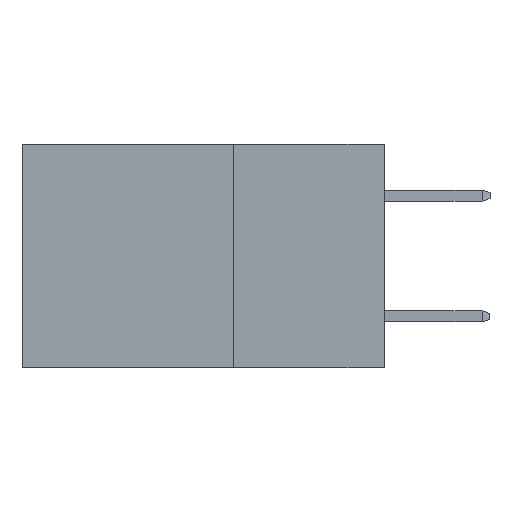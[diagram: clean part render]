
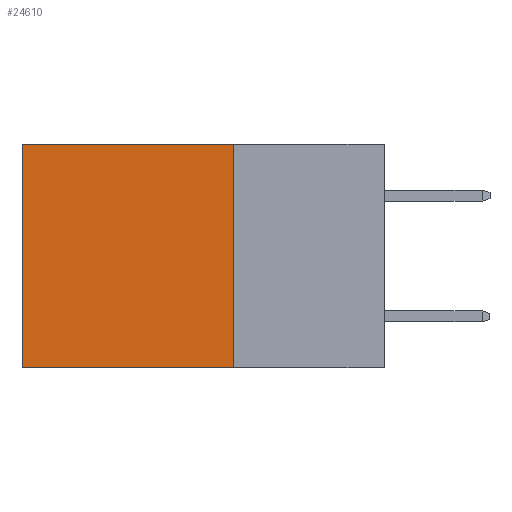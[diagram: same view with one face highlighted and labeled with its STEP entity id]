
A CAD part, left-side view. The second image highlights one B-rep face of the part: STEP entity #24610.
In plain terms, the highlighted planar face has unit normal (-1, 0, 0).
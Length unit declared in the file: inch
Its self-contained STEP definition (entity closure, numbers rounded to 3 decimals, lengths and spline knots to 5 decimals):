
#1134 = VERTEX_POINT ( 'NONE', #25334 ) ;
#1688 = CARTESIAN_POINT ( 'NONE',  ( 0.298, 0.25, -0.37 ) ) ;
#2410 = CARTESIAN_POINT ( 'NONE',  ( 0.298, 0.6, -0.37 ) ) ;
#3016 = CARTESIAN_POINT ( 'NONE',  ( 0.298, 0.25, 0. ) ) ;
#3137 = EDGE_CURVE ( 'NONE', #9688, #5686, #3156, .T. ) ;
#3156 = LINE ( 'NONE', #22431, #15515 ) ;
#4174 = DIRECTION ( 'NONE',  ( 0., 1., 0. ) ) ;
#5402 = CARTESIAN_POINT ( 'NONE',  ( 0.298, 0.25, -0.37 ) ) ;
#5686 = VERTEX_POINT ( 'NONE', #5402 ) ;
#6096 = LINE ( 'NONE', #1688, #24787 ) ;
#6149 = ORIENTED_EDGE ( 'NONE', *, *, #23729, .T. ) ;
#6759 = CARTESIAN_POINT ( 'NONE',  ( 0.298, 0.6, 0. ) ) ;
#8873 = ORIENTED_EDGE ( 'NONE', *, *, #27057, .F. ) ;
#9224 = DIRECTION ( 'NONE',  ( 0., 0., -1. ) ) ;
#9688 = VERTEX_POINT ( 'NONE', #17093 ) ;
#9778 = DIRECTION ( 'NONE',  ( 0., 1., 0. ) ) ;
#10498 = AXIS2_PLACEMENT_3D ( 'NONE', #3016, #12986, #29750 ) ;
#10506 = PLANE ( 'NONE',  #10498 ) ;
#11254 = VECTOR ( 'NONE', #9224, 39.37008 ) ;
#12671 = VERTEX_POINT ( 'NONE', #2410 ) ;
#12986 = DIRECTION ( 'NONE',  ( 1., 0., 0. ) ) ;
#15515 = VECTOR ( 'NONE', #19076, 39.37008 ) ;
#15983 = VECTOR ( 'NONE', #9778, 39.37008 ) ;
#17093 = CARTESIAN_POINT ( 'NONE',  ( 0.298, 0.25, 0. ) ) ;
#17289 = EDGE_CURVE ( 'NONE', #1134, #12671, #23424, .T. ) ;
#19076 = DIRECTION ( 'NONE',  ( 0., 0., -1. ) ) ;
#21591 = FACE_OUTER_BOUND ( 'NONE', #21893, .T. ) ;
#21893 = EDGE_LOOP ( 'NONE', ( #30359, #8873, #24408, #6149 ) ) ;
#22431 = CARTESIAN_POINT ( 'NONE',  ( 0.298, 0.25, 0. ) ) ;
#23424 = LINE ( 'NONE', #6759, #11254 ) ;
#23729 = EDGE_CURVE ( 'NONE', #9688, #1134, #28722, .T. ) ;
#24408 = ORIENTED_EDGE ( 'NONE', *, *, #3137, .F. ) ;
#24610 = ADVANCED_FACE ( 'NONE', ( #21591 ), #10506, .F. ) ;
#24787 = VECTOR ( 'NONE', #4174, 39.37008 ) ;
#25334 = CARTESIAN_POINT ( 'NONE',  ( 0.298, 0.6, 0. ) ) ;
#27057 = EDGE_CURVE ( 'NONE', #5686, #12671, #6096, .T. ) ;
#27179 = CARTESIAN_POINT ( 'NONE',  ( 0.298, 0.25, 0. ) ) ;
#28722 = LINE ( 'NONE', #27179, #15983 ) ;
#29750 = DIRECTION ( 'NONE',  ( 0., 0., -1. ) ) ;
#30359 = ORIENTED_EDGE ( 'NONE', *, *, #17289, .T. ) ;
